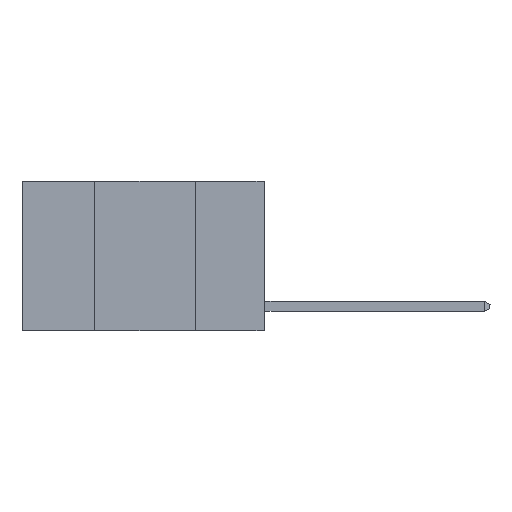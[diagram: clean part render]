
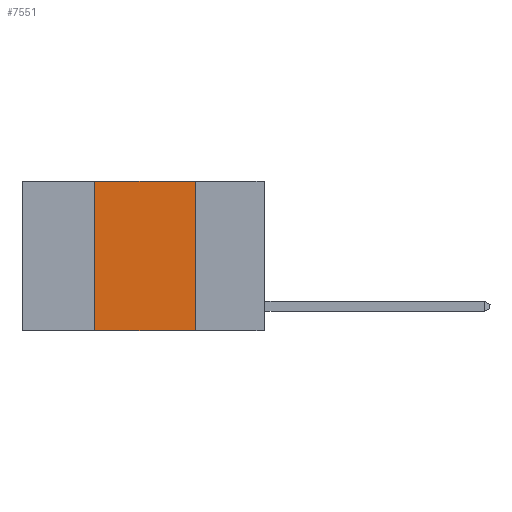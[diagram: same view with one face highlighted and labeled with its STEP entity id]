
A CAD part, left-side view. The second image highlights one B-rep face of the part: STEP entity #7551.
In plain terms, the highlighted planar face has unit normal (-1, 0, 0).
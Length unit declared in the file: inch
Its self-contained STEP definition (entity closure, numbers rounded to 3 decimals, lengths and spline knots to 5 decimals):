
#607 = CARTESIAN_POINT ( 'NONE',  ( 0., 0.17, -0.37 ) ) ;
#1457 = EDGE_CURVE ( 'NONE', #6750, #12011, #12907, .T. ) ;
#1814 = VECTOR ( 'NONE', #10763, 39.37008 ) ;
#2550 = CARTESIAN_POINT ( 'NONE',  ( 0., 0.17, 0. ) ) ;
#2684 = CARTESIAN_POINT ( 'NONE',  ( 0., 0.42, -0.37 ) ) ;
#3093 = VECTOR ( 'NONE', #11548, 39.37008 ) ;
#5599 = VECTOR ( 'NONE', #14053, 39.37008 ) ;
#5863 = CARTESIAN_POINT ( 'NONE',  ( 0., 0.42, 0. ) ) ;
#5997 = VERTEX_POINT ( 'NONE', #13376 ) ;
#6096 = FACE_OUTER_BOUND ( 'NONE', #11111, .T. ) ;
#6750 = VERTEX_POINT ( 'NONE', #2684 ) ;
#6754 = LINE ( 'NONE', #14265, #3093 ) ;
#7098 = AXIS2_PLACEMENT_3D ( 'NONE', #15298, #16634, #8537 ) ;
#7551 = ADVANCED_FACE ( 'NONE', ( #6096 ), #16577, .F. ) ;
#7687 = ORIENTED_EDGE ( 'NONE', *, *, #11929, .T. ) ;
#8180 = ORIENTED_EDGE ( 'NONE', *, *, #1457, .F. ) ;
#8537 = DIRECTION ( 'NONE',  ( 0., 0., -1. ) ) ;
#9421 = CARTESIAN_POINT ( 'NONE',  ( 0., 0.6, -0.37 ) ) ;
#9543 = LINE ( 'NONE', #2550, #1814 ) ;
#10763 = DIRECTION ( 'NONE',  ( 0., 0., -1. ) ) ;
#11111 = EDGE_LOOP ( 'NONE', ( #16279, #14666, #8180, #7687 ) ) ;
#11548 = DIRECTION ( 'NONE',  ( 0., -1., 0. ) ) ;
#11643 = VERTEX_POINT ( 'NONE', #607 ) ;
#11929 = EDGE_CURVE ( 'NONE', #6750, #11643, #15531, .T. ) ;
#12009 = VECTOR ( 'NONE', #13574, 39.37008 ) ;
#12011 = VERTEX_POINT ( 'NONE', #12395 ) ;
#12395 = CARTESIAN_POINT ( 'NONE',  ( 0., 0.42, 0. ) ) ;
#12907 = LINE ( 'NONE', #5863, #5599 ) ;
#13376 = CARTESIAN_POINT ( 'NONE',  ( 0., 0.17, 0. ) ) ;
#13564 = EDGE_CURVE ( 'NONE', #5997, #11643, #9543, .T. ) ;
#13574 = DIRECTION ( 'NONE',  ( 0., -1., 0. ) ) ;
#13909 = EDGE_CURVE ( 'NONE', #12011, #5997, #6754, .T. ) ;
#14053 = DIRECTION ( 'NONE',  ( 0., 0., 1. ) ) ;
#14265 = CARTESIAN_POINT ( 'NONE',  ( 0., 0.6, 0. ) ) ;
#14666 = ORIENTED_EDGE ( 'NONE', *, *, #13909, .F. ) ;
#15298 = CARTESIAN_POINT ( 'NONE',  ( 0., 0.6, 0. ) ) ;
#15531 = LINE ( 'NONE', #9421, #12009 ) ;
#16279 = ORIENTED_EDGE ( 'NONE', *, *, #13564, .F. ) ;
#16577 = PLANE ( 'NONE',  #7098 ) ;
#16634 = DIRECTION ( 'NONE',  ( 1., 0., 0. ) ) ;
